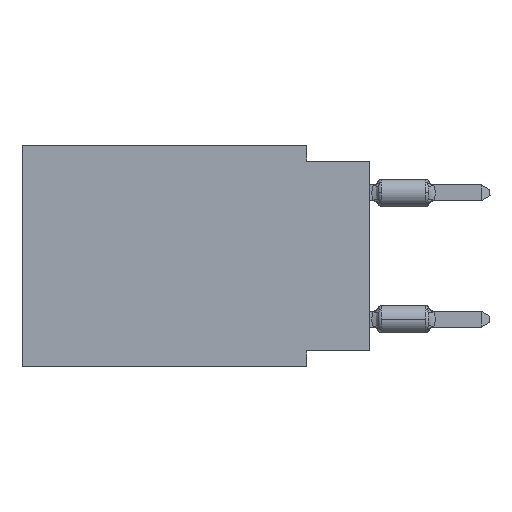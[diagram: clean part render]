
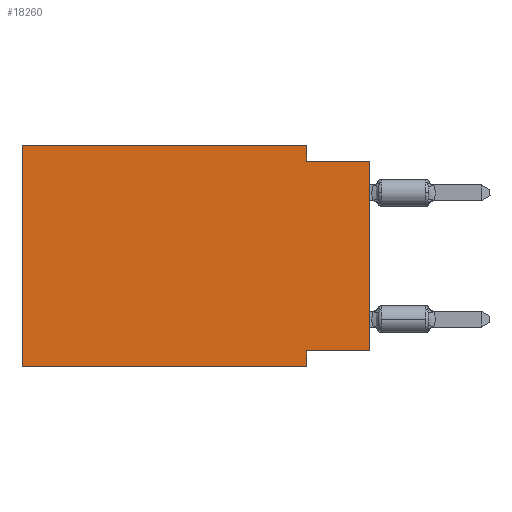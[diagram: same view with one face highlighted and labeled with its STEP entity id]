
A CAD part, left-side view. The second image highlights one B-rep face of the part: STEP entity #18260.
In plain terms, the highlighted planar face has unit normal (-1, 0, 0).
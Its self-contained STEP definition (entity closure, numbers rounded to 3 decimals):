
#267 = VECTOR ( 'NONE', #22683, 1000. ) ;
#1612 = ORIENTED_EDGE ( 'NONE', *, *, #36311, .T. ) ;
#3295 = VERTEX_POINT ( 'NONE', #38236 ) ;
#4325 = EDGE_LOOP ( 'NONE', ( #28671, #39923, #32944, #33908, #38908, #1612, #22506, #5418 ) ) ;
#4805 = VECTOR ( 'NONE', #46719, 1000. ) ;
#5418 = ORIENTED_EDGE ( 'NONE', *, *, #5560, .F. ) ;
#5472 = LINE ( 'NONE', #47531, #4805 ) ;
#5560 = EDGE_CURVE ( 'NONE', #19087, #7095, #41942, .T. ) ;
#6249 = DIRECTION ( 'NONE',  ( 0., 0., -1. ) ) ;
#6426 = DIRECTION ( 'NONE',  ( 0., 0., -1. ) ) ;
#6960 = FACE_OUTER_BOUND ( 'NONE', #4325, .T. ) ;
#7095 = VERTEX_POINT ( 'NONE', #12344 ) ;
#8892 = EDGE_CURVE ( 'NONE', #39304, #48416, #36340, .T. ) ;
#9111 = CARTESIAN_POINT ( 'NONE',  ( 0., 0., -8.255 ) ) ;
#10384 = CARTESIAN_POINT ( 'NONE',  ( 0., 13.97, -8.89 ) ) ;
#10711 = VECTOR ( 'NONE', #22061, 1000. ) ;
#11297 = CARTESIAN_POINT ( 'NONE',  ( 0., 13.97, 0. ) ) ;
#12344 = CARTESIAN_POINT ( 'NONE',  ( 0., 2.54, -8.255 ) ) ;
#13810 = VECTOR ( 'NONE', #52971, 1000. ) ;
#14625 = LINE ( 'NONE', #47728, #29984 ) ;
#15029 = CARTESIAN_POINT ( 'NONE',  ( 0., 2.54, -0.635 ) ) ;
#15162 = DIRECTION ( 'NONE',  ( 0., 0., 1. ) ) ;
#15607 = CARTESIAN_POINT ( 'NONE',  ( 0., 0., -0.635 ) ) ;
#15996 = EDGE_CURVE ( 'NONE', #7095, #51094, #5472, .T. ) ;
#16611 = EDGE_CURVE ( 'NONE', #19087, #22317, #14625, .T. ) ;
#17199 = CARTESIAN_POINT ( 'NONE',  ( 0., 2.54, 0. ) ) ;
#18260 = ADVANCED_FACE ( 'NONE', ( #6960 ), #44677, .F. ) ;
#19073 = VECTOR ( 'NONE', #21326, 1000. ) ;
#19087 = VERTEX_POINT ( 'NONE', #22789 ) ;
#20410 = EDGE_CURVE ( 'NONE', #3295, #50822, #47812, .T. ) ;
#20627 = AXIS2_PLACEMENT_3D ( 'NONE', #11297, #24067, #6426 ) ;
#21326 = DIRECTION ( 'NONE',  ( 0., 1., 0. ) ) ;
#22061 = DIRECTION ( 'NONE',  ( 0., -1., 0. ) ) ;
#22124 = CARTESIAN_POINT ( 'NONE',  ( 0., 2.54, -8.89 ) ) ;
#22317 = VERTEX_POINT ( 'NONE', #25628 ) ;
#22506 = ORIENTED_EDGE ( 'NONE', *, *, #15996, .F. ) ;
#22609 = LINE ( 'NONE', #10384, #10711 ) ;
#22683 = DIRECTION ( 'NONE',  ( 0., -1., 0. ) ) ;
#22789 = CARTESIAN_POINT ( 'NONE',  ( 0., 0., -8.255 ) ) ;
#22961 = LINE ( 'NONE', #15607, #267 ) ;
#23678 = DIRECTION ( 'NONE',  ( 0., -1., 0. ) ) ;
#24067 = DIRECTION ( 'NONE',  ( 1., 0., 0. ) ) ;
#25628 = CARTESIAN_POINT ( 'NONE',  ( 0., 0., -0.635 ) ) ;
#27160 = CARTESIAN_POINT ( 'NONE',  ( 0., 2.54, 0. ) ) ;
#28671 = ORIENTED_EDGE ( 'NONE', *, *, #16611, .T. ) ;
#29146 = EDGE_CURVE ( 'NONE', #48416, #22317, #22961, .T. ) ;
#29984 = VECTOR ( 'NONE', #15162, 1000. ) ;
#32944 = ORIENTED_EDGE ( 'NONE', *, *, #8892, .F. ) ;
#33908 = ORIENTED_EDGE ( 'NONE', *, *, #37877, .F. ) ;
#34209 = VECTOR ( 'NONE', #23678, 1000. ) ;
#36311 = EDGE_CURVE ( 'NONE', #3295, #51094, #22609, .T. ) ;
#36340 = LINE ( 'NONE', #27160, #46191 ) ;
#37877 = EDGE_CURVE ( 'NONE', #50822, #39304, #40762, .T. ) ;
#38236 = CARTESIAN_POINT ( 'NONE',  ( 0., 13.97, -8.89 ) ) ;
#38908 = ORIENTED_EDGE ( 'NONE', *, *, #20410, .F. ) ;
#39304 = VERTEX_POINT ( 'NONE', #17199 ) ;
#39923 = ORIENTED_EDGE ( 'NONE', *, *, #29146, .F. ) ;
#40762 = LINE ( 'NONE', #53524, #34209 ) ;
#41942 = LINE ( 'NONE', #9111, #19073 ) ;
#42794 = CARTESIAN_POINT ( 'NONE',  ( 0., 13.97, 0. ) ) ;
#44677 = PLANE ( 'NONE',  #20627 ) ;
#46191 = VECTOR ( 'NONE', #6249, 1000. ) ;
#46719 = DIRECTION ( 'NONE',  ( 0., 0., -1. ) ) ;
#47531 = CARTESIAN_POINT ( 'NONE',  ( 0., 2.54, -8.89 ) ) ;
#47728 = CARTESIAN_POINT ( 'NONE',  ( 0., 0., 0. ) ) ;
#47812 = LINE ( 'NONE', #48350, #13810 ) ;
#48350 = CARTESIAN_POINT ( 'NONE',  ( 0., 13.97, 0. ) ) ;
#48416 = VERTEX_POINT ( 'NONE', #15029 ) ;
#50822 = VERTEX_POINT ( 'NONE', #42794 ) ;
#51094 = VERTEX_POINT ( 'NONE', #22124 ) ;
#52971 = DIRECTION ( 'NONE',  ( 0., 0., 1. ) ) ;
#53524 = CARTESIAN_POINT ( 'NONE',  ( 0., 13.97, 0. ) ) ;
